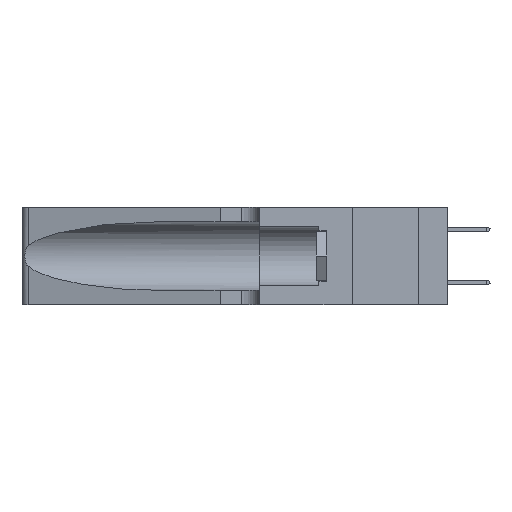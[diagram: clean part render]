
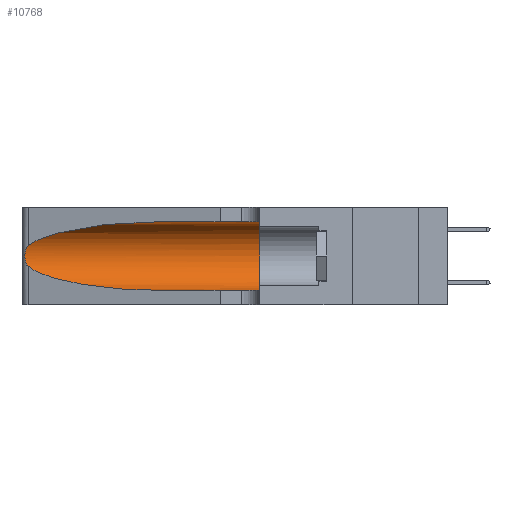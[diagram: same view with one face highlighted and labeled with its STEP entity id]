
A CAD part, left-side view. The second image highlights one B-rep face of the part: STEP entity #10768.
In plain terms, the highlighted cylindrical face has radius 3.308 mm (diameter 6.617 mm), a partial arc.
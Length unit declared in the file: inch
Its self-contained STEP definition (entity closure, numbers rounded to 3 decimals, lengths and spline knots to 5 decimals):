
#267 = CARTESIAN_POINT ( 'NONE',  ( 0.26018, 1.23835, 0.19895 ) ) ;
#275 = CARTESIAN_POINT ( 'NONE',  ( 0.1305, 0.72297, 0.05475 ) ) ;
#574 = CARTESIAN_POINT ( 'NONE',  ( 0.1305, 1.61858, 0.31525 ) ) ;
#1670 = VERTEX_POINT ( 'NONE', #28437 ) ;
#2480 = CARTESIAN_POINT ( 'NONE',  ( 0.25487, 1.22718, 0.14631 ) ) ;
#2573 = CARTESIAN_POINT ( 'NONE',  ( 0.26075, 1.23896, 0.178 ) ) ;
#2883 = FACE_OUTER_BOUND ( 'NONE', #9111, .T. ) ;
#3470 = ORIENTED_EDGE ( 'NONE', *, *, #13557, .T. ) ;
#4154 = LINE ( 'NONE', #574, #27658 ) ;
#4888 = CARTESIAN_POINT ( 'NONE',  ( 0.25856, 1.23593, 0.16098 ) ) ;
#5586 = EDGE_CURVE ( 'NONE', #10619, #1670, #26255, .T. ) ;
#6276 = CARTESIAN_POINT ( 'NONE',  ( 0.2373, 1.15595, 0.28018 ) ) ;
#7088 = CARTESIAN_POINT ( 'NONE',  ( 0.25555, 1.22994, 0.2215 ) ) ;
#7185 = CARTESIAN_POINT ( 'NONE',  ( 0.25639, 1.23186, 0.15144 ) ) ;
#7488 = DIRECTION ( 'NONE',  ( 0., -1., 0. ) ) ;
#7964 = ORIENTED_EDGE ( 'NONE', *, *, #22344, .T. ) ;
#9111 = EDGE_LOOP ( 'NONE', ( #7964, #24089, #22170, #3470, #11786, #13778 ) ) ;
#9486 = CARTESIAN_POINT ( 'NONE',  ( 0.25487, 1.22718, 0.14631 ) ) ;
#10051 =( BOUNDED_CURVE ( )  B_SPLINE_CURVE ( 3, ( #17660, #22146, #6276, #22247 ),
 .UNSPECIFIED., .F., .F. ) 
 B_SPLINE_CURVE_WITH_KNOTS ( ( 4, 4 ),
 ( 1.5708, 2.84003 ),
 .UNSPECIFIED. ) 
 CURVE ( )  GEOMETRIC_REPRESENTATION_ITEM ( )  RATIONAL_B_SPLINE_CURVE ( ( 1., 0.87, 0.87, 1. ) ) 
 REPRESENTATION_ITEM ( '' )  );
#10153 = CARTESIAN_POINT ( 'NONE',  ( 0.1305, 0.35, 0.185 ) ) ;
#10619 = VERTEX_POINT ( 'NONE', #21597 ) ;
#10768 = ADVANCED_FACE ( 'NONE', ( #2883 ), #20409, .F. ) ;
#11621 = CARTESIAN_POINT ( 'NONE',  ( 0.2373, 1.15595, 0.08982 ) ) ;
#11715 = CARTESIAN_POINT ( 'NONE',  ( 0.25639, 1.23184, 0.21858 ) ) ;
#11786 = ORIENTED_EDGE ( 'NONE', *, *, #18153, .F. ) ;
#11934 = AXIS2_PLACEMENT_3D ( 'NONE', #15306, #24447, #19902 ) ;
#12469 = DIRECTION ( 'NONE',  ( 0., 0., 1. ) ) ;
#12813 = CARTESIAN_POINT ( 'NONE',  ( 0.1305, 0.72297, 0.31525 ) ) ;
#13043 = VERTEX_POINT ( 'NONE', #25210 ) ;
#13557 = EDGE_CURVE ( 'NONE', #1670, #13043, #23301, .T. ) ;
#13778 = ORIENTED_EDGE ( 'NONE', *, *, #23860, .F. ) ;
#13814 = VERTEX_POINT ( 'NONE', #25360 ) ;
#14003 = CARTESIAN_POINT ( 'NONE',  ( 0.25854, 1.2359, 0.20912 ) ) ;
#14007 = CARTESIAN_POINT ( 'NONE',  ( 0.18966, 0.96281, 0.05475 ) ) ;
#15306 = CARTESIAN_POINT ( 'NONE',  ( 0.1305, 1.61858, 0.185 ) ) ;
#15597 = VERTEX_POINT ( 'NONE', #20432 ) ;
#16287 = CARTESIAN_POINT ( 'NONE',  ( 0.26075, 1.23896, 0.19203 ) ) ;
#16516 = VECTOR ( 'NONE', #29008, 39.37008 ) ;
#17195 = AXIS2_PLACEMENT_3D ( 'NONE', #10153, #26054, #12469 ) ;
#17660 = CARTESIAN_POINT ( 'NONE',  ( 0.1305, 0.72297, 0.31525 ) ) ;
#18153 = EDGE_CURVE ( 'NONE', #13814, #13043, #18426, .T. ) ;
#18426 = CIRCLE ( 'NONE', #17195, 0.13025 ) ;
#18584 = CARTESIAN_POINT ( 'NONE',  ( 0.26017, 1.23833, 0.17102 ) ) ;
#18765 = B_SPLINE_CURVE_WITH_KNOTS ( 'NONE', 3,
 ( #23072, #7088, #11715, #27564, #14003, #267, #16287, #2573, #18584, #4888, #20891, #7185, #23164, #9486 ),
 .UNSPECIFIED., .F., .F.,
 ( 4, 2, 2, 2, 2, 2, 4 ),
 ( 0., 0.00027, 0.00053, 0.00107, 0.0016, 0.00187, 0.00214 ),
 .UNSPECIFIED. ) ;
#19902 = DIRECTION ( 'NONE',  ( 0., 0., -1. ) ) ;
#19943 = CARTESIAN_POINT ( 'NONE',  ( 0.1305, 1.61858, 0.05475 ) ) ;
#20409 = CYLINDRICAL_SURFACE ( 'NONE', #11934, 0.13025 ) ;
#20432 = CARTESIAN_POINT ( 'NONE',  ( 0.25487, 1.22718, 0.22369 ) ) ;
#20566 = EDGE_CURVE ( 'NONE', #15597, #10619, #18765, .T. ) ;
#20891 = CARTESIAN_POINT ( 'NONE',  ( 0.25789, 1.23486, 0.15765 ) ) ;
#21597 = CARTESIAN_POINT ( 'NONE',  ( 0.25487, 1.22718, 0.14631 ) ) ;
#22146 = CARTESIAN_POINT ( 'NONE',  ( 0.18966, 0.96281, 0.31525 ) ) ;
#22170 = ORIENTED_EDGE ( 'NONE', *, *, #5586, .T. ) ;
#22247 = CARTESIAN_POINT ( 'NONE',  ( 0.25487, 1.22718, 0.22369 ) ) ;
#22344 = EDGE_CURVE ( 'NONE', #26148, #15597, #10051, .T. ) ;
#23072 = CARTESIAN_POINT ( 'NONE',  ( 0.25487, 1.22718, 0.22369 ) ) ;
#23164 = CARTESIAN_POINT ( 'NONE',  ( 0.25555, 1.22993, 0.14849 ) ) ;
#23301 = LINE ( 'NONE', #19943, #16516 ) ;
#23860 = EDGE_CURVE ( 'NONE', #26148, #13814, #4154, .T. ) ;
#24089 = ORIENTED_EDGE ( 'NONE', *, *, #20566, .T. ) ;
#24447 = DIRECTION ( 'NONE',  ( 0., -1., 0. ) ) ;
#25210 = CARTESIAN_POINT ( 'NONE',  ( 0.1305, 0.35, 0.05475 ) ) ;
#25360 = CARTESIAN_POINT ( 'NONE',  ( 0.1305, 0.35, 0.31525 ) ) ;
#26054 = DIRECTION ( 'NONE',  ( 0., 1., 0. ) ) ;
#26148 = VERTEX_POINT ( 'NONE', #12813 ) ;
#26255 =( BOUNDED_CURVE ( )  B_SPLINE_CURVE ( 3, ( #2480, #11621, #14007, #275 ),
 .UNSPECIFIED., .F., .T. ) 
 B_SPLINE_CURVE_WITH_KNOTS ( ( 4, 4 ),
 ( 3.44316, 4.71239 ),
 .UNSPECIFIED. ) 
 CURVE ( )  GEOMETRIC_REPRESENTATION_ITEM ( )  RATIONAL_B_SPLINE_CURVE ( ( 1., 0.87, 0.87, 1. ) ) 
 REPRESENTATION_ITEM ( '' )  );
#27564 = CARTESIAN_POINT ( 'NONE',  ( 0.25787, 1.23484, 0.2124 ) ) ;
#27658 = VECTOR ( 'NONE', #7488, 39.37008 ) ;
#28437 = CARTESIAN_POINT ( 'NONE',  ( 0.1305, 0.72297, 0.05475 ) ) ;
#29008 = DIRECTION ( 'NONE',  ( 0., -1., 0. ) ) ;
